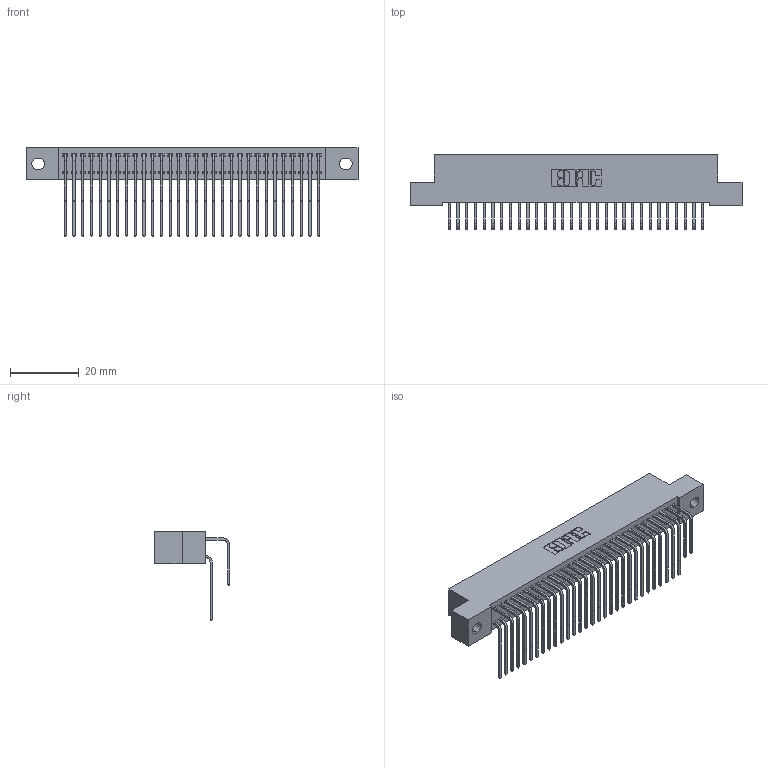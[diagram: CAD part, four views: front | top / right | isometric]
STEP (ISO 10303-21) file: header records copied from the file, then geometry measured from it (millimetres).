
FILE_DESCRIPTION (( 'STEP AP203' ), '1' );
FILE_NAME ('392-060-558-202.STEP', '2019-10-08T17:35:11', ( '' ), ( '' ), 'SwSTEP 2.0', 'SolidWorks 2016', '' );
FILE_SCHEMA (( 'CONFIG_CONTROL_DESIGN' ));
Length unit declared in the file: inch
Products named in the file (4): 342 Part_.128 Slot; 345-292-001_558 559 Tail - 1; 345-292-001_558 Tail - 2; 392-060-558-202
Assembly tree (61 placements, depth 2):
  392-060-558-202
    342 Part_.128 Slot
    345-292-001_558 559 Tail - 1  x30
    345-292-001_558 Tail - 2  x30
Bounding box: 96.52 x 21.91 x 25.78 mm (x, y, z)
Volume: 8909.5 mm3; surface area: 15532 mm2
Topology: 61 solids, 61 shells, 3354 faces, 9971 edges, 6566 vertices
Faces by surface type: plane 2350, cylinder 1004
Entity records: 22639 total; most frequent: CARTESIAN_POINT 3817, ORIENTED_EDGE 3702, DIRECTION 3263, EDGE_CURVE 1851, VECTOR 1683, LINE 1683, VERTEX_POINT 1230, AXIS2_PLACEMENT_3D 790
